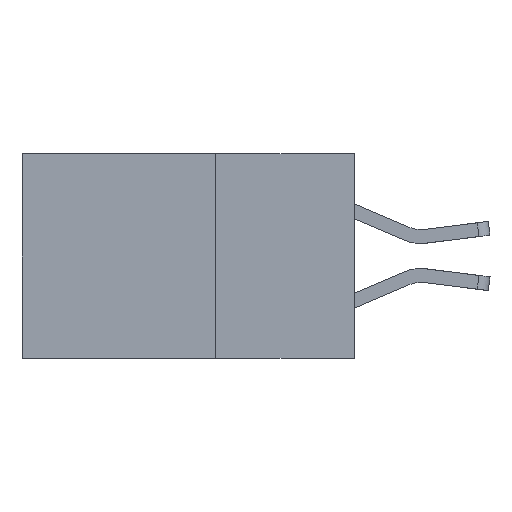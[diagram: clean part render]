
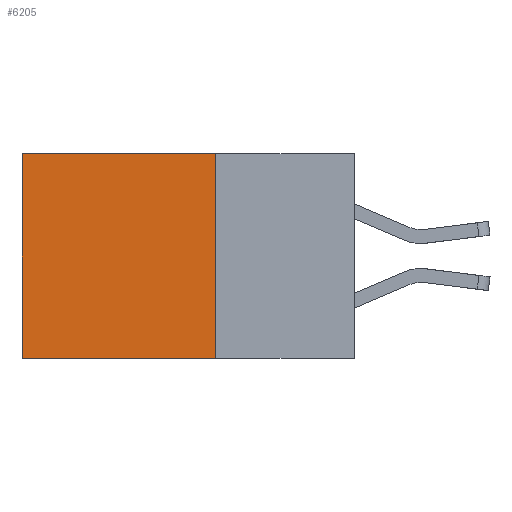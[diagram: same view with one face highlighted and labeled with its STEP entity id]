
A CAD part, left-side view. The second image highlights one B-rep face of the part: STEP entity #6205.
In plain terms, the highlighted planar face has unit normal (-1, 0, 0).
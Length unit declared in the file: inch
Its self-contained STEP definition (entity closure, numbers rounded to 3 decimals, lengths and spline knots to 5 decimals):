
#763 = ORIENTED_EDGE ( 'NONE', *, *, #1910, .F. ) ;
#1166 = DIRECTION ( 'NONE',  ( 0., 0., -1. ) ) ;
#1328 = ORIENTED_EDGE ( 'NONE', *, *, #10293, .T. ) ;
#1377 = VERTEX_POINT ( 'NONE', #9003 ) ;
#1438 = DIRECTION ( 'NONE',  ( 1., 0., 0. ) ) ;
#1530 = VECTOR ( 'NONE', #6346, 39.37008 ) ;
#1910 = EDGE_CURVE ( 'NONE', #3178, #1377, #10426, .T. ) ;
#2335 = DIRECTION ( 'NONE',  ( 0., 1., 0. ) ) ;
#3178 = VERTEX_POINT ( 'NONE', #9384 ) ;
#3692 = VERTEX_POINT ( 'NONE', #7623 ) ;
#3949 = ORIENTED_EDGE ( 'NONE', *, *, #5289, .T. ) ;
#4399 = FACE_OUTER_BOUND ( 'NONE', #6683, .T. ) ;
#5289 = EDGE_CURVE ( 'NONE', #5561, #3692, #6921, .T. ) ;
#5485 = CARTESIAN_POINT ( 'NONE',  ( 0.2615, 0.25, -0.37 ) ) ;
#5561 = VERTEX_POINT ( 'NONE', #6454 ) ;
#6098 = ORIENTED_EDGE ( 'NONE', *, *, #6286, .F. ) ;
#6205 = ADVANCED_FACE ( 'NONE', ( #4399 ), #6408, .F. ) ;
#6286 = EDGE_CURVE ( 'NONE', #1377, #3692, #8019, .T. ) ;
#6346 = DIRECTION ( 'NONE',  ( 0., 0., -1. ) ) ;
#6357 = CARTESIAN_POINT ( 'NONE',  ( 0.2615, 0.25, -0.37 ) ) ;
#6408 = PLANE ( 'NONE',  #10247 ) ;
#6454 = CARTESIAN_POINT ( 'NONE',  ( 0.2615, 0.6, 0. ) ) ;
#6683 = EDGE_LOOP ( 'NONE', ( #3949, #6098, #763, #1328 ) ) ;
#6921 = LINE ( 'NONE', #6954, #8297 ) ;
#6954 = CARTESIAN_POINT ( 'NONE',  ( 0.2615, 0.6, -0.37 ) ) ;
#7218 = DIRECTION ( 'NONE',  ( 0., 0., -1. ) ) ;
#7623 = CARTESIAN_POINT ( 'NONE',  ( 0.2615, 0.6, -0.37 ) ) ;
#7741 = VECTOR ( 'NONE', #8858, 39.37008 ) ;
#7988 = LINE ( 'NONE', #8053, #7741 ) ;
#8019 = LINE ( 'NONE', #10414, #10354 ) ;
#8053 = CARTESIAN_POINT ( 'NONE',  ( 0.2615, 0.25, 0. ) ) ;
#8297 = VECTOR ( 'NONE', #1166, 39.37008 ) ;
#8858 = DIRECTION ( 'NONE',  ( 0., 1., 0. ) ) ;
#9003 = CARTESIAN_POINT ( 'NONE',  ( 0.2615, 0.25, -0.37 ) ) ;
#9384 = CARTESIAN_POINT ( 'NONE',  ( 0.2615, 0.25, 0. ) ) ;
#10247 = AXIS2_PLACEMENT_3D ( 'NONE', #5485, #1438, #7218 ) ;
#10293 = EDGE_CURVE ( 'NONE', #3178, #5561, #7988, .T. ) ;
#10354 = VECTOR ( 'NONE', #2335, 39.37008 ) ;
#10414 = CARTESIAN_POINT ( 'NONE',  ( 0.2615, 0.25, -0.37 ) ) ;
#10426 = LINE ( 'NONE', #6357, #1530 ) ;
